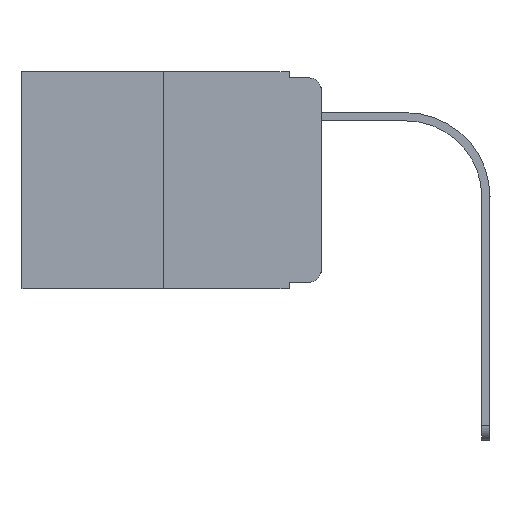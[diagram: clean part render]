
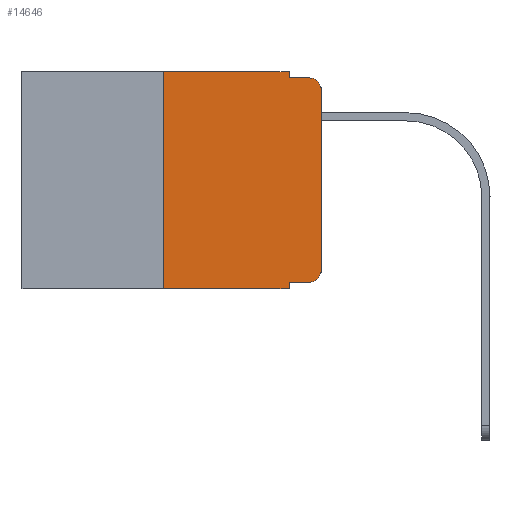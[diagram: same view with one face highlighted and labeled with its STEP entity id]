
A CAD part, left-side view. The second image highlights one B-rep face of the part: STEP entity #14646.
In plain terms, the highlighted planar face has unit normal (-1, 0, 0).
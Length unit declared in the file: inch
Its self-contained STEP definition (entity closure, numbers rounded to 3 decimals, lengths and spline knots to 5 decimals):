
#737 = CARTESIAN_POINT ( 'NONE',  ( 0., 0.051, 0. ) ) ;
#935 = CARTESIAN_POINT ( 'NONE',  ( 0., 0.25, 0. ) ) ;
#1087 = CARTESIAN_POINT ( 'NONE',  ( 0., 0., -0.313 ) ) ;
#1096 = EDGE_CURVE ( 'NONE', #3232, #1984, #3853, .T. ) ;
#1111 = CARTESIAN_POINT ( 'NONE',  ( 0., 0.051, -0.343 ) ) ;
#1205 = EDGE_CURVE ( 'NONE', #7818, #3129, #3131, .T. ) ;
#1258 = CARTESIAN_POINT ( 'NONE',  ( 0., 0.02, -0.333 ) ) ;
#1458 = DIRECTION ( 'NONE',  ( 0., 0., -1. ) ) ;
#1640 = CARTESIAN_POINT ( 'NONE',  ( 0., 0.25, -0.343 ) ) ;
#1659 = VECTOR ( 'NONE', #9657, 39.37008 ) ;
#1940 = EDGE_CURVE ( 'NONE', #11698, #7818, #10069, .T. ) ;
#1984 = VERTEX_POINT ( 'NONE', #1258 ) ;
#2490 = VERTEX_POINT ( 'NONE', #1111 ) ;
#3129 = VERTEX_POINT ( 'NONE', #6667 ) ;
#3131 = LINE ( 'NONE', #11177, #1659 ) ;
#3232 = VERTEX_POINT ( 'NONE', #12407 ) ;
#3600 = DIRECTION ( 'NONE',  ( 0., 0., -1. ) ) ;
#3759 = AXIS2_PLACEMENT_3D ( 'NONE', #11900, #10573, #3600 ) ;
#3853 = LINE ( 'NONE', #13561, #16066 ) ;
#4094 = CARTESIAN_POINT ( 'NONE',  ( 0., 0.02, -0.01 ) ) ;
#4111 = EDGE_CURVE ( 'NONE', #11533, #11698, #8955, .T. ) ;
#4334 = VECTOR ( 'NONE', #5563, 39.37008 ) ;
#4363 = VERTEX_POINT ( 'NONE', #4094 ) ;
#4701 = EDGE_CURVE ( 'NONE', #3129, #4363, #14852, .T. ) ;
#5438 = CIRCLE ( 'NONE', #3759, 0.02 ) ;
#5563 = DIRECTION ( 'NONE',  ( 0., -1., 0. ) ) ;
#5589 = LINE ( 'NONE', #9397, #15075 ) ;
#5699 = EDGE_CURVE ( 'NONE', #14984, #10801, #14147, .T. ) ;
#5769 = ORIENTED_EDGE ( 'NONE', *, *, #9325, .T. ) ;
#6076 = ORIENTED_EDGE ( 'NONE', *, *, #4701, .F. ) ;
#6452 = LINE ( 'NONE', #6880, #4334 ) ;
#6581 = AXIS2_PLACEMENT_3D ( 'NONE', #11053, #6657, #13200 ) ;
#6657 = DIRECTION ( 'NONE',  ( 1., 0., 0. ) ) ;
#6667 = CARTESIAN_POINT ( 'NONE',  ( 0., 0.051, -0.01 ) ) ;
#6765 = ORIENTED_EDGE ( 'NONE', *, *, #5699, .T. ) ;
#6880 = CARTESIAN_POINT ( 'NONE',  ( 0., 0.473, -0.343 ) ) ;
#7058 = FACE_OUTER_BOUND ( 'NONE', #7661, .T. ) ;
#7102 = VECTOR ( 'NONE', #14358, 39.37008 ) ;
#7221 = DIRECTION ( 'NONE',  ( -1., 0., 0. ) ) ;
#7303 = VECTOR ( 'NONE', #15310, 39.37008 ) ;
#7496 = DIRECTION ( 'NONE',  ( 0., 0., -1. ) ) ;
#7661 = EDGE_LOOP ( 'NONE', ( #6765, #14103, #6076, #14039, #9280, #11359, #5769, #10806, #11030, #13281 ) ) ;
#7775 = CARTESIAN_POINT ( 'NONE',  ( 0., 0.473, 0. ) ) ;
#7818 = VERTEX_POINT ( 'NONE', #737 ) ;
#8042 = CARTESIAN_POINT ( 'NONE',  ( 0., 0.051, -0.01 ) ) ;
#8223 = EDGE_CURVE ( 'NONE', #1984, #14984, #11073, .T. ) ;
#8521 = VECTOR ( 'NONE', #16363, 39.37008 ) ;
#8645 = CARTESIAN_POINT ( 'NONE',  ( 0., 0.02, -0.313 ) ) ;
#8955 = LINE ( 'NONE', #935, #7102 ) ;
#9240 = DIRECTION ( 'NONE',  ( 0., -1., 0. ) ) ;
#9280 = ORIENTED_EDGE ( 'NONE', *, *, #1940, .F. ) ;
#9325 = EDGE_CURVE ( 'NONE', #11533, #2490, #6452, .T. ) ;
#9397 = CARTESIAN_POINT ( 'NONE',  ( 0., 0.051, 0. ) ) ;
#9657 = DIRECTION ( 'NONE',  ( 0., 0., -1. ) ) ;
#10069 = LINE ( 'NONE', #7775, #13651 ) ;
#10107 = EDGE_CURVE ( 'NONE', #10801, #4363, #5438, .T. ) ;
#10198 = CARTESIAN_POINT ( 'NONE',  ( 0., 0.25, 0. ) ) ;
#10427 = DIRECTION ( 'NONE',  ( 0., -1., 0. ) ) ;
#10573 = DIRECTION ( 'NONE',  ( -1., 0., 0. ) ) ;
#10801 = VERTEX_POINT ( 'NONE', #16835 ) ;
#10806 = ORIENTED_EDGE ( 'NONE', *, *, #13045, .F. ) ;
#11030 = ORIENTED_EDGE ( 'NONE', *, *, #1096, .T. ) ;
#11053 = CARTESIAN_POINT ( 'NONE',  ( 0., 0.473, 0. ) ) ;
#11073 = CIRCLE ( 'NONE', #15916, 0.02 ) ;
#11177 = CARTESIAN_POINT ( 'NONE',  ( 0., 0.051, 0. ) ) ;
#11359 = ORIENTED_EDGE ( 'NONE', *, *, #4111, .F. ) ;
#11533 = VERTEX_POINT ( 'NONE', #1640 ) ;
#11698 = VERTEX_POINT ( 'NONE', #10198 ) ;
#11900 = CARTESIAN_POINT ( 'NONE',  ( 0., 0.02, -0.03 ) ) ;
#12407 = CARTESIAN_POINT ( 'NONE',  ( 0., 0.051, -0.333 ) ) ;
#13045 = EDGE_CURVE ( 'NONE', #3232, #2490, #5589, .T. ) ;
#13200 = DIRECTION ( 'NONE',  ( 0., 0., -1. ) ) ;
#13281 = ORIENTED_EDGE ( 'NONE', *, *, #8223, .T. ) ;
#13561 = CARTESIAN_POINT ( 'NONE',  ( 0., 0.051, -0.333 ) ) ;
#13651 = VECTOR ( 'NONE', #10427, 39.37008 ) ;
#14039 = ORIENTED_EDGE ( 'NONE', *, *, #1205, .F. ) ;
#14103 = ORIENTED_EDGE ( 'NONE', *, *, #10107, .T. ) ;
#14147 = LINE ( 'NONE', #16746, #7303 ) ;
#14358 = DIRECTION ( 'NONE',  ( 0., 0., 1. ) ) ;
#14641 = PLANE ( 'NONE',  #6581 ) ;
#14646 = ADVANCED_FACE ( 'NONE', ( #7058 ), #14641, .F. ) ;
#14852 = LINE ( 'NONE', #8042, #8521 ) ;
#14984 = VERTEX_POINT ( 'NONE', #1087 ) ;
#15075 = VECTOR ( 'NONE', #1458, 39.37008 ) ;
#15310 = DIRECTION ( 'NONE',  ( 0., 0., 1. ) ) ;
#15916 = AXIS2_PLACEMENT_3D ( 'NONE', #8645, #7221, #7496 ) ;
#16066 = VECTOR ( 'NONE', #9240, 39.37008 ) ;
#16363 = DIRECTION ( 'NONE',  ( 0., -1., 0. ) ) ;
#16746 = CARTESIAN_POINT ( 'NONE',  ( 0., 0., 0. ) ) ;
#16835 = CARTESIAN_POINT ( 'NONE',  ( 0., 0., -0.03 ) ) ;
